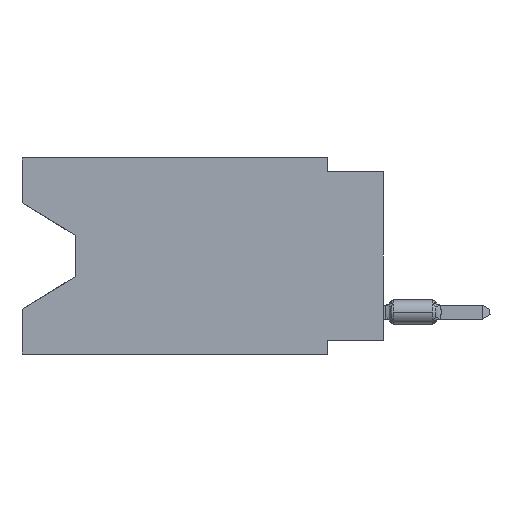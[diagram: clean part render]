
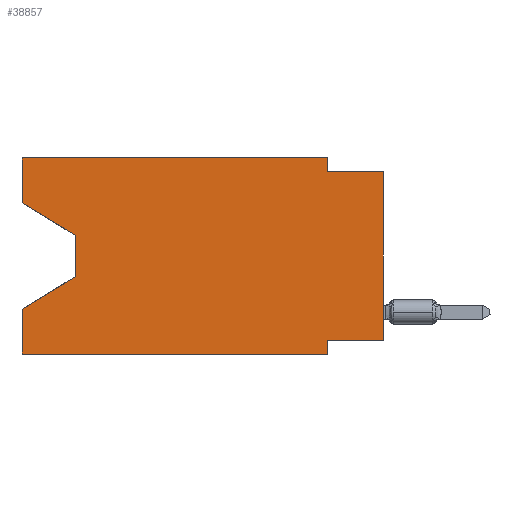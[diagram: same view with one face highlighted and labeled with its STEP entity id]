
A CAD part, left-side view. The second image highlights one B-rep face of the part: STEP entity #38857.
In plain terms, the highlighted planar face has unit normal (-1, 0, 0).
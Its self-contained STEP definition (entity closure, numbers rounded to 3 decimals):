
#900 = CARTESIAN_POINT ( 'NONE',  ( 0., 0., 0. ) ) ;
#904 = LINE ( 'NONE', #103486, #107452 ) ;
#1312 = ORIENTED_EDGE ( 'NONE', *, *, #73937, .T. ) ;
#2535 = DIRECTION ( 'NONE',  ( 1., 0., 0. ) ) ;
#4742 = VECTOR ( 'NONE', #62100, 1000. ) ;
#5054 = ORIENTED_EDGE ( 'NONE', *, *, #28449, .T. ) ;
#5742 = DIRECTION ( 'NONE',  ( 0., 0., -1. ) ) ;
#6750 = DIRECTION ( 'NONE',  ( 0., 0., -1. ) ) ;
#10394 = DIRECTION ( 'NONE',  ( 0., 0., -1. ) ) ;
#10657 = VECTOR ( 'NONE', #55211, 1000. ) ;
#10923 = VECTOR ( 'NONE', #94889, 1000. ) ;
#12339 = VERTEX_POINT ( 'NONE', #68213 ) ;
#17337 = LINE ( 'NONE', #81898, #76429 ) ;
#19459 = CARTESIAN_POINT ( 'NONE',  ( 0., 16.383, 0. ) ) ;
#20934 = VERTEX_POINT ( 'NONE', #83570 ) ;
#20965 = DIRECTION ( 'NONE',  ( 0., -1., 0. ) ) ;
#21263 = CARTESIAN_POINT ( 'NONE',  ( 0., 0., -8.255 ) ) ;
#22419 = ORIENTED_EDGE ( 'NONE', *, *, #80838, .F. ) ;
#23936 = DIRECTION ( 'NONE',  ( 0., -1., 0. ) ) ;
#25394 = VERTEX_POINT ( 'NONE', #42706 ) ;
#25938 = ORIENTED_EDGE ( 'NONE', *, *, #77963, .F. ) ;
#26492 = LINE ( 'NONE', #71182, #4742 ) ;
#26824 = ORIENTED_EDGE ( 'NONE', *, *, #65185, .F. ) ;
#27050 = ORIENTED_EDGE ( 'NONE', *, *, #62971, .F. ) ;
#27208 = CARTESIAN_POINT ( 'NONE',  ( 0., 2.54, -8.89 ) ) ;
#28449 = EDGE_CURVE ( 'NONE', #33807, #67974, #39991, .T. ) ;
#30077 = VERTEX_POINT ( 'NONE', #76689 ) ;
#33807 = VERTEX_POINT ( 'NONE', #67609 ) ;
#34069 = CARTESIAN_POINT ( 'NONE',  ( 0., 2.54, 0. ) ) ;
#38857 = ADVANCED_FACE ( 'NONE', ( #39944 ), #103947, .F. ) ;
#39944 = FACE_OUTER_BOUND ( 'NONE', #76922, .T. ) ;
#39991 = LINE ( 'NONE', #114803, #101819 ) ;
#40027 = EDGE_CURVE ( 'NONE', #58884, #100165, #76780, .T. ) ;
#41235 = DIRECTION ( 'NONE',  ( 0., 0., 1. ) ) ;
#41934 = LINE ( 'NONE', #34069, #58579 ) ;
#42706 = CARTESIAN_POINT ( 'NONE',  ( 0., 13.97, -3.505 ) ) ;
#45581 = CARTESIAN_POINT ( 'NONE',  ( 0., 16.383, -8.89 ) ) ;
#46646 = LINE ( 'NONE', #54513, #57104 ) ;
#47922 = EDGE_CURVE ( 'NONE', #12339, #116070, #85539, .T. ) ;
#48287 = DIRECTION ( 'NONE',  ( 0., -0.855, -0.519 ) ) ;
#51274 = ORIENTED_EDGE ( 'NONE', *, *, #88903, .T. ) ;
#54513 = CARTESIAN_POINT ( 'NONE',  ( 0., 16.383, 0. ) ) ;
#55211 = DIRECTION ( 'NONE',  ( 0., 0., 1. ) ) ;
#57104 = VECTOR ( 'NONE', #91944, 1000. ) ;
#58579 = VECTOR ( 'NONE', #5742, 1000. ) ;
#58884 = VERTEX_POINT ( 'NONE', #72600 ) ;
#59317 = CARTESIAN_POINT ( 'NONE',  ( 0., 16.383, 0. ) ) ;
#61933 = EDGE_CURVE ( 'NONE', #58884, #20934, #93226, .T. ) ;
#62100 = DIRECTION ( 'NONE',  ( 0., 0., -1. ) ) ;
#62971 = EDGE_CURVE ( 'NONE', #30077, #20934, #113859, .T. ) ;
#65185 = EDGE_CURVE ( 'NONE', #100165, #97086, #91214, .T. ) ;
#65740 = CARTESIAN_POINT ( 'NONE',  ( 0., 16.383, -6.852 ) ) ;
#66406 = AXIS2_PLACEMENT_3D ( 'NONE', #19459, #2535, #10394 ) ;
#66973 = CARTESIAN_POINT ( 'NONE',  ( 0., 16.383, -2.038 ) ) ;
#67421 = CARTESIAN_POINT ( 'NONE',  ( 0., 16.383, 0. ) ) ;
#67609 = CARTESIAN_POINT ( 'NONE',  ( 0., 13.97, -5.385 ) ) ;
#67974 = VERTEX_POINT ( 'NONE', #65740 ) ;
#68213 = CARTESIAN_POINT ( 'NONE',  ( 0., 16.383, 0. ) ) ;
#70186 = LINE ( 'NONE', #59317, #92844 ) ;
#71066 = VECTOR ( 'NONE', #6750, 1000. ) ;
#71182 = CARTESIAN_POINT ( 'NONE',  ( 0., 13.97, -3.505 ) ) ;
#71224 = VECTOR ( 'NONE', #20965, 1000. ) ;
#72149 = ORIENTED_EDGE ( 'NONE', *, *, #95784, .F. ) ;
#72241 = CARTESIAN_POINT ( 'NONE',  ( 0., 2.54, -8.255 ) ) ;
#72600 = CARTESIAN_POINT ( 'NONE',  ( 0., 0., -8.255 ) ) ;
#73937 = EDGE_CURVE ( 'NONE', #25394, #33807, #26492, .T. ) ;
#76429 = VECTOR ( 'NONE', #118699, 1000. ) ;
#76689 = CARTESIAN_POINT ( 'NONE',  ( 0., 2.54, -0.635 ) ) ;
#76780 = LINE ( 'NONE', #21263, #10923 ) ;
#76922 = EDGE_LOOP ( 'NONE', ( #51274, #1312, #5054, #22419, #80755, #26824, #118541, #90581, #27050, #25938, #114722, #72149 ) ) ;
#77963 = EDGE_CURVE ( 'NONE', #116070, #30077, #41934, .T. ) ;
#80206 = VECTOR ( 'NONE', #23936, 1000. ) ;
#80629 = EDGE_CURVE ( 'NONE', #108321, #97086, #17337, .T. ) ;
#80755 = ORIENTED_EDGE ( 'NONE', *, *, #80629, .T. ) ;
#80838 = EDGE_CURVE ( 'NONE', #108321, #67974, #46646, .T. ) ;
#81898 = CARTESIAN_POINT ( 'NONE',  ( 0., 16.383, -8.89 ) ) ;
#83570 = CARTESIAN_POINT ( 'NONE',  ( 0., 0., -0.635 ) ) ;
#85539 = LINE ( 'NONE', #67421, #71224 ) ;
#87121 = VERTEX_POINT ( 'NONE', #66973 ) ;
#88903 = EDGE_CURVE ( 'NONE', #87121, #25394, #904, .T. ) ;
#89432 = CARTESIAN_POINT ( 'NONE',  ( 0., 2.54, -8.89 ) ) ;
#90581 = ORIENTED_EDGE ( 'NONE', *, *, #61933, .T. ) ;
#91214 = LINE ( 'NONE', #89432, #71066 ) ;
#91944 = DIRECTION ( 'NONE',  ( 0., 0., 1. ) ) ;
#92844 = VECTOR ( 'NONE', #41235, 1000. ) ;
#93226 = LINE ( 'NONE', #900, #10657 ) ;
#94889 = DIRECTION ( 'NONE',  ( 0., 1., 0. ) ) ;
#95522 = DIRECTION ( 'NONE',  ( 0., 0.855, -0.519 ) ) ;
#95784 = EDGE_CURVE ( 'NONE', #87121, #12339, #70186, .T. ) ;
#96373 = CARTESIAN_POINT ( 'NONE',  ( 0., 0., -0.635 ) ) ;
#97086 = VERTEX_POINT ( 'NONE', #27208 ) ;
#97563 = CARTESIAN_POINT ( 'NONE',  ( 0., 2.54, 0. ) ) ;
#100165 = VERTEX_POINT ( 'NONE', #72241 ) ;
#101819 = VECTOR ( 'NONE', #95522, 1000. ) ;
#103486 = CARTESIAN_POINT ( 'NONE',  ( 0., 16.383, -2.038 ) ) ;
#103947 = PLANE ( 'NONE',  #66406 ) ;
#107452 = VECTOR ( 'NONE', #48287, 1000. ) ;
#108321 = VERTEX_POINT ( 'NONE', #45581 ) ;
#113859 = LINE ( 'NONE', #96373, #80206 ) ;
#114722 = ORIENTED_EDGE ( 'NONE', *, *, #47922, .F. ) ;
#114803 = CARTESIAN_POINT ( 'NONE',  ( 0., 13.97, -5.385 ) ) ;
#116070 = VERTEX_POINT ( 'NONE', #97563 ) ;
#118541 = ORIENTED_EDGE ( 'NONE', *, *, #40027, .F. ) ;
#118699 = DIRECTION ( 'NONE',  ( 0., -1., 0. ) ) ;
